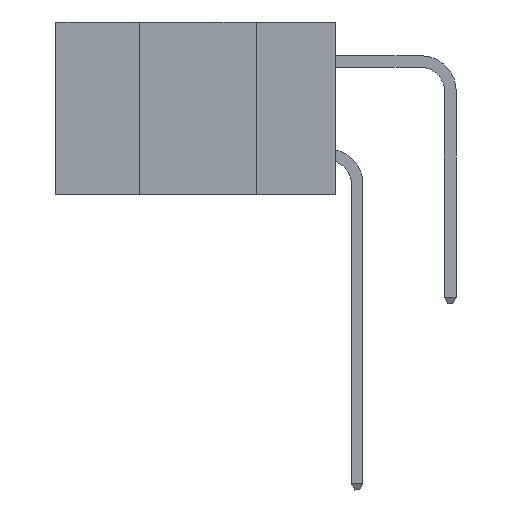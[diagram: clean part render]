
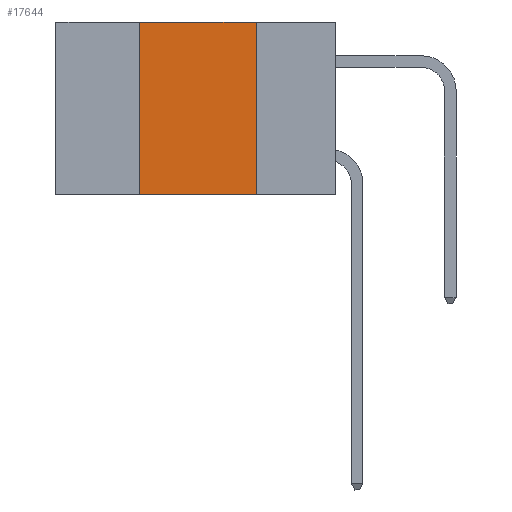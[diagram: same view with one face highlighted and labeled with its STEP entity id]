
A CAD part, left-side view. The second image highlights one B-rep face of the part: STEP entity #17644.
In plain terms, the highlighted planar face has unit normal (-1, 0, 0).
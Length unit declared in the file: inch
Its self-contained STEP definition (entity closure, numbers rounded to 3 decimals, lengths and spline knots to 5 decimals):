
#207 = DIRECTION ( 'NONE',  ( 0., 0., -1. ) ) ;
#1596 = DIRECTION ( 'NONE',  ( 0., -1., 0. ) ) ;
#2328 = DIRECTION ( 'NONE',  ( 1., 0., 0. ) ) ;
#2693 = FACE_OUTER_BOUND ( 'NONE', #23152, .T. ) ;
#4189 = EDGE_CURVE ( 'NONE', #28947, #9775, #11996, .T. ) ;
#4529 = AXIS2_PLACEMENT_3D ( 'NONE', #32399, #2328, #207 ) ;
#4612 = EDGE_CURVE ( 'NONE', #28947, #15997, #15690, .T. ) ;
#4979 = ORIENTED_EDGE ( 'NONE', *, *, #4612, .F. ) ;
#6976 = CARTESIAN_POINT ( 'NONE',  ( 0., 0.42, -0.37 ) ) ;
#9775 = VERTEX_POINT ( 'NONE', #16622 ) ;
#10020 = DIRECTION ( 'NONE',  ( 0., -1., 0. ) ) ;
#11996 = LINE ( 'NONE', #12855, #27878 ) ;
#12855 = CARTESIAN_POINT ( 'NONE',  ( 0., 0.6, -0.37 ) ) ;
#14336 = CARTESIAN_POINT ( 'NONE',  ( 0., 0.42, 0. ) ) ;
#14863 = VECTOR ( 'NONE', #31530, 39.37008 ) ;
#15690 = LINE ( 'NONE', #32410, #25994 ) ;
#15997 = VERTEX_POINT ( 'NONE', #14336 ) ;
#16622 = CARTESIAN_POINT ( 'NONE',  ( 0., 0.17, -0.37 ) ) ;
#17644 = ADVANCED_FACE ( 'NONE', ( #2693 ), #29075, .F. ) ;
#17762 = EDGE_CURVE ( 'NONE', #27441, #9775, #32593, .T. ) ;
#19349 = CARTESIAN_POINT ( 'NONE',  ( 0., 0.17, 0. ) ) ;
#19423 = ORIENTED_EDGE ( 'NONE', *, *, #4189, .T. ) ;
#20597 = VECTOR ( 'NONE', #10020, 39.37008 ) ;
#21874 = CARTESIAN_POINT ( 'NONE',  ( 0., 0.6, 0. ) ) ;
#23152 = EDGE_LOOP ( 'NONE', ( #25049, #35711, #4979, #19423 ) ) ;
#24561 = EDGE_CURVE ( 'NONE', #15997, #27441, #26660, .T. ) ;
#25049 = ORIENTED_EDGE ( 'NONE', *, *, #17762, .F. ) ;
#25994 = VECTOR ( 'NONE', #32276, 39.37008 ) ;
#26660 = LINE ( 'NONE', #21874, #20597 ) ;
#27441 = VERTEX_POINT ( 'NONE', #28052 ) ;
#27878 = VECTOR ( 'NONE', #1596, 39.37008 ) ;
#28052 = CARTESIAN_POINT ( 'NONE',  ( 0., 0.17, 0. ) ) ;
#28947 = VERTEX_POINT ( 'NONE', #6976 ) ;
#29075 = PLANE ( 'NONE',  #4529 ) ;
#31530 = DIRECTION ( 'NONE',  ( 0., 0., -1. ) ) ;
#32276 = DIRECTION ( 'NONE',  ( 0., 0., 1. ) ) ;
#32399 = CARTESIAN_POINT ( 'NONE',  ( 0., 0.6, 0. ) ) ;
#32410 = CARTESIAN_POINT ( 'NONE',  ( 0., 0.42, 0. ) ) ;
#32593 = LINE ( 'NONE', #19349, #14863 ) ;
#35711 = ORIENTED_EDGE ( 'NONE', *, *, #24561, .F. ) ;
